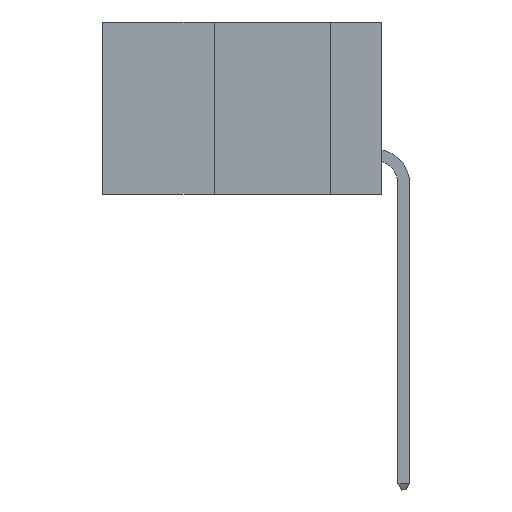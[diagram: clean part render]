
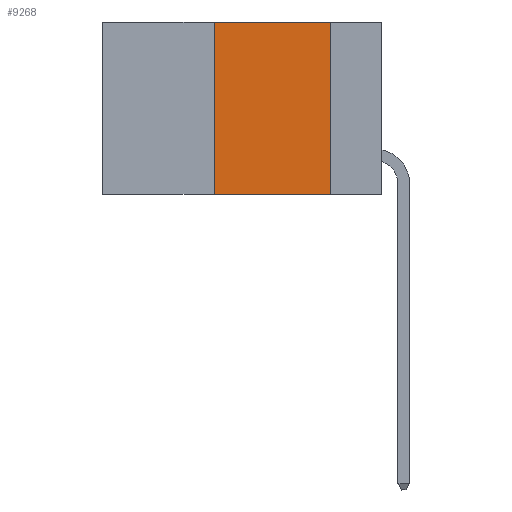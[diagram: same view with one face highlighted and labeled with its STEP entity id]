
A CAD part, left-side view. The second image highlights one B-rep face of the part: STEP entity #9268.
In plain terms, the highlighted planar face has unit normal (-1, 0, 0).
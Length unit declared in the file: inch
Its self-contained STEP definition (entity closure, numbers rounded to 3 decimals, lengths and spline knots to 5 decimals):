
#144 = ORIENTED_EDGE ( 'NONE', *, *, #5624, .T. ) ;
#190 = VERTEX_POINT ( 'NONE', #6561 ) ;
#227 = DIRECTION ( 'NONE',  ( 0., 0., 1. ) ) ;
#467 = CARTESIAN_POINT ( 'NONE',  ( 0., 0.6, -0.37 ) ) ;
#1683 = CARTESIAN_POINT ( 'NONE',  ( 0., 0.6, 0. ) ) ;
#1850 = EDGE_LOOP ( 'NONE', ( #8527, #7481, #7464, #144 ) ) ;
#1907 = LINE ( 'NONE', #467, #3244 ) ;
#1935 = LINE ( 'NONE', #6179, #6241 ) ;
#2048 = CARTESIAN_POINT ( 'NONE',  ( 0., 0.11, 0. ) ) ;
#2520 = FACE_OUTER_BOUND ( 'NONE', #1850, .T. ) ;
#2631 = CARTESIAN_POINT ( 'NONE',  ( 0., 0.6, 0. ) ) ;
#2798 = EDGE_CURVE ( 'NONE', #3616, #3108, #7822, .T. ) ;
#3047 = VECTOR ( 'NONE', #7899, 39.37008 ) ;
#3108 = VERTEX_POINT ( 'NONE', #2048 ) ;
#3244 = VECTOR ( 'NONE', #9167, 39.37008 ) ;
#3512 = LINE ( 'NONE', #9728, #5339 ) ;
#3616 = VERTEX_POINT ( 'NONE', #4708 ) ;
#3786 = DIRECTION ( 'NONE',  ( 0., 0., -1. ) ) ;
#4708 = CARTESIAN_POINT ( 'NONE',  ( 0., 0.36, 0. ) ) ;
#4898 = PLANE ( 'NONE',  #9226 ) ;
#5113 = DIRECTION ( 'NONE',  ( 1., 0., 0. ) ) ;
#5339 = VECTOR ( 'NONE', #227, 39.37008 ) ;
#5624 = EDGE_CURVE ( 'NONE', #8773, #190, #1907, .T. ) ;
#5940 = CARTESIAN_POINT ( 'NONE',  ( 0., 0.36, -0.37 ) ) ;
#6179 = CARTESIAN_POINT ( 'NONE',  ( 0., 0.11, 0. ) ) ;
#6241 = VECTOR ( 'NONE', #3786, 39.37008 ) ;
#6561 = CARTESIAN_POINT ( 'NONE',  ( 0., 0.11, -0.37 ) ) ;
#6574 = DIRECTION ( 'NONE',  ( 0., 0., -1. ) ) ;
#7464 = ORIENTED_EDGE ( 'NONE', *, *, #9854, .F. ) ;
#7481 = ORIENTED_EDGE ( 'NONE', *, *, #2798, .F. ) ;
#7822 = LINE ( 'NONE', #1683, #3047 ) ;
#7899 = DIRECTION ( 'NONE',  ( 0., -1., 0. ) ) ;
#8527 = ORIENTED_EDGE ( 'NONE', *, *, #8843, .F. ) ;
#8773 = VERTEX_POINT ( 'NONE', #5940 ) ;
#8843 = EDGE_CURVE ( 'NONE', #3108, #190, #1935, .T. ) ;
#9167 = DIRECTION ( 'NONE',  ( 0., -1., 0. ) ) ;
#9226 = AXIS2_PLACEMENT_3D ( 'NONE', #2631, #5113, #6574 ) ;
#9268 = ADVANCED_FACE ( 'NONE', ( #2520 ), #4898, .F. ) ;
#9728 = CARTESIAN_POINT ( 'NONE',  ( 0., 0.36, 0. ) ) ;
#9854 = EDGE_CURVE ( 'NONE', #8773, #3616, #3512, .T. ) ;
